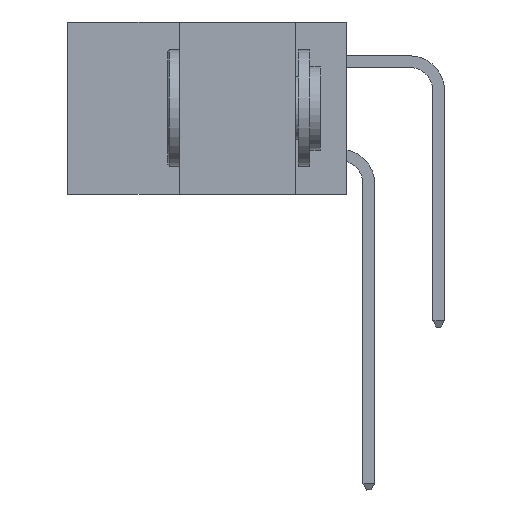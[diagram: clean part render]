
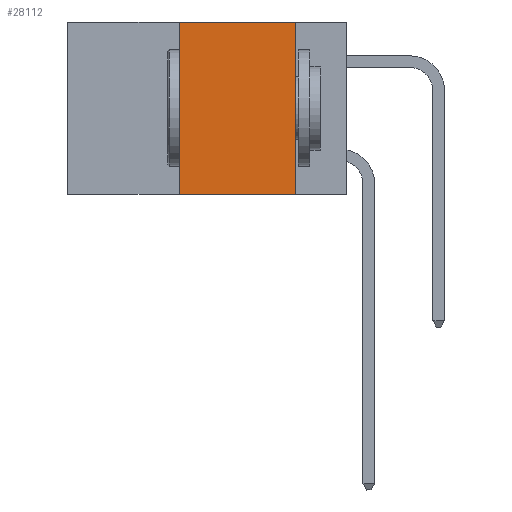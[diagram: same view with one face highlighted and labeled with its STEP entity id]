
A CAD part, left-side view. The second image highlights one B-rep face of the part: STEP entity #28112.
In plain terms, the highlighted planar face has unit normal (-1, 0, 0).
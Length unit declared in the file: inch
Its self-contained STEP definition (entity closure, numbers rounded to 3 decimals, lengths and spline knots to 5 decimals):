
#2163 = DIRECTION ( 'NONE',  ( 1., 0., 0. ) ) ;
#4318 = DIRECTION ( 'NONE',  ( 0., 0., -1. ) ) ;
#4422 = CARTESIAN_POINT ( 'NONE',  ( 0., 0.6, 0. ) ) ;
#4760 = LINE ( 'NONE', #29595, #10617 ) ;
#6828 = CARTESIAN_POINT ( 'NONE',  ( 0., 0.36, 0. ) ) ;
#7233 = CARTESIAN_POINT ( 'NONE',  ( 0., 0.36, -0.37 ) ) ;
#7501 = AXIS2_PLACEMENT_3D ( 'NONE', #4422, #2163, #22351 ) ;
#8577 = CARTESIAN_POINT ( 'NONE',  ( 0., 0.6, 0. ) ) ;
#8944 = ORIENTED_EDGE ( 'NONE', *, *, #13003, .F. ) ;
#9012 = CARTESIAN_POINT ( 'NONE',  ( 0., 0.11, -0.37 ) ) ;
#9658 = LINE ( 'NONE', #30390, #32300 ) ;
#9747 = EDGE_CURVE ( 'NONE', #26792, #27996, #9658, .T. ) ;
#9938 = DIRECTION ( 'NONE',  ( 0., -1., 0. ) ) ;
#10617 = VECTOR ( 'NONE', #4318, 39.37008 ) ;
#11258 = FACE_OUTER_BOUND ( 'NONE', #26638, .T. ) ;
#11483 = VECTOR ( 'NONE', #13562, 39.37008 ) ;
#11808 = CARTESIAN_POINT ( 'NONE',  ( 0., 0.11, 0. ) ) ;
#13003 = EDGE_CURVE ( 'NONE', #14992, #22870, #4760, .T. ) ;
#13562 = DIRECTION ( 'NONE',  ( 0., -1., 0. ) ) ;
#14271 = CARTESIAN_POINT ( 'NONE',  ( 0., 0.6, -0.37 ) ) ;
#14992 = VERTEX_POINT ( 'NONE', #11808 ) ;
#15137 = LINE ( 'NONE', #14271, #31412 ) ;
#22351 = DIRECTION ( 'NONE',  ( 0., 0., -1. ) ) ;
#22566 = PLANE ( 'NONE',  #7501 ) ;
#22870 = VERTEX_POINT ( 'NONE', #9012 ) ;
#24101 = EDGE_CURVE ( 'NONE', #26792, #22870, #15137, .T. ) ;
#25277 = DIRECTION ( 'NONE',  ( 0., 0., 1. ) ) ;
#25836 = EDGE_CURVE ( 'NONE', #27996, #14992, #29761, .T. ) ;
#26638 = EDGE_LOOP ( 'NONE', ( #8944, #31394, #31708, #30006 ) ) ;
#26792 = VERTEX_POINT ( 'NONE', #7233 ) ;
#27996 = VERTEX_POINT ( 'NONE', #6828 ) ;
#28112 = ADVANCED_FACE ( 'NONE', ( #11258 ), #22566, .F. ) ;
#29595 = CARTESIAN_POINT ( 'NONE',  ( 0., 0.11, 0. ) ) ;
#29761 = LINE ( 'NONE', #8577, #11483 ) ;
#30006 = ORIENTED_EDGE ( 'NONE', *, *, #24101, .T. ) ;
#30390 = CARTESIAN_POINT ( 'NONE',  ( 0., 0.36, 0. ) ) ;
#31394 = ORIENTED_EDGE ( 'NONE', *, *, #25836, .F. ) ;
#31412 = VECTOR ( 'NONE', #9938, 39.37008 ) ;
#31708 = ORIENTED_EDGE ( 'NONE', *, *, #9747, .F. ) ;
#32300 = VECTOR ( 'NONE', #25277, 39.37008 ) ;
